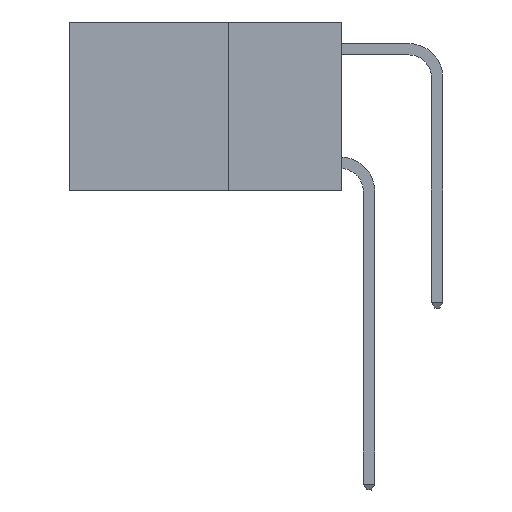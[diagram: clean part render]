
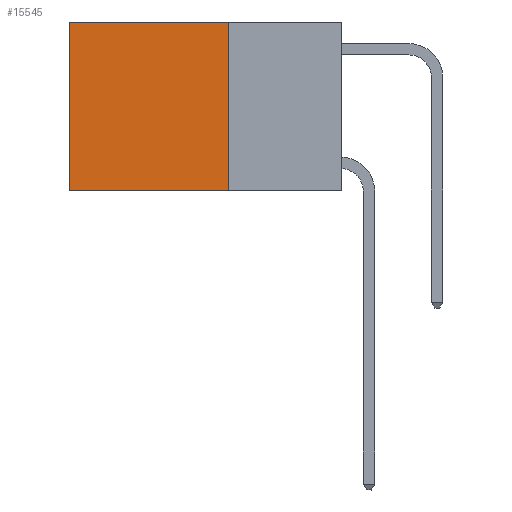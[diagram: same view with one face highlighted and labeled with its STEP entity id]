
A CAD part, left-side view. The second image highlights one B-rep face of the part: STEP entity #15545.
In plain terms, the highlighted planar face has unit normal (-1, 0, 0).
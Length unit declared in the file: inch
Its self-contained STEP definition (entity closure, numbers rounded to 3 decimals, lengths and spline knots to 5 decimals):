
#1530 = VECTOR ( 'NONE', #3508, 39.37008 ) ;
#3508 = DIRECTION ( 'NONE',  ( 0., 0., -1. ) ) ;
#3874 = EDGE_CURVE ( 'NONE', #4207, #9457, #12296, .T. ) ;
#4207 = VERTEX_POINT ( 'NONE', #15103 ) ;
#5973 = CARTESIAN_POINT ( 'NONE',  ( 0.2625, 0.25, 0. ) ) ;
#6600 = AXIS2_PLACEMENT_3D ( 'NONE', #9775, #12023, #27789 ) ;
#6822 = CARTESIAN_POINT ( 'NONE',  ( 0.2625, 0.6, 0. ) ) ;
#8485 = FACE_OUTER_BOUND ( 'NONE', #18595, .T. ) ;
#9457 = VERTEX_POINT ( 'NONE', #6822 ) ;
#9775 = CARTESIAN_POINT ( 'NONE',  ( 0.2625, 0.25, 0. ) ) ;
#10378 = EDGE_CURVE ( 'NONE', #9457, #12412, #19596, .T. ) ;
#10769 = LINE ( 'NONE', #23659, #15364 ) ;
#11673 = CARTESIAN_POINT ( 'NONE',  ( 0.2625, 0.25, 0. ) ) ;
#12023 = DIRECTION ( 'NONE',  ( 1., 0., 0. ) ) ;
#12296 = LINE ( 'NONE', #11673, #24304 ) ;
#12398 = ORIENTED_EDGE ( 'NONE', *, *, #13010, .F. ) ;
#12408 = DIRECTION ( 'NONE',  ( 0., 1., 0. ) ) ;
#12412 = VERTEX_POINT ( 'NONE', #19362 ) ;
#13010 = EDGE_CURVE ( 'NONE', #18789, #12412, #10769, .T. ) ;
#13878 = ORIENTED_EDGE ( 'NONE', *, *, #18491, .F. ) ;
#15103 = CARTESIAN_POINT ( 'NONE',  ( 0.2625, 0.25, 0. ) ) ;
#15364 = VECTOR ( 'NONE', #12408, 39.37008 ) ;
#15545 = ADVANCED_FACE ( 'NONE', ( #8485 ), #23289, .F. ) ;
#18491 = EDGE_CURVE ( 'NONE', #4207, #18789, #22839, .T. ) ;
#18595 = EDGE_LOOP ( 'NONE', ( #27157, #12398, #13878, #22835 ) ) ;
#18789 = VERTEX_POINT ( 'NONE', #22736 ) ;
#19362 = CARTESIAN_POINT ( 'NONE',  ( 0.2625, 0.6, -0.37 ) ) ;
#19596 = LINE ( 'NONE', #28246, #1530 ) ;
#21783 = DIRECTION ( 'NONE',  ( 0., 0., -1. ) ) ;
#22736 = CARTESIAN_POINT ( 'NONE',  ( 0.2625, 0.25, -0.37 ) ) ;
#22835 = ORIENTED_EDGE ( 'NONE', *, *, #3874, .T. ) ;
#22839 = LINE ( 'NONE', #5973, #28087 ) ;
#23289 = PLANE ( 'NONE',  #6600 ) ;
#23659 = CARTESIAN_POINT ( 'NONE',  ( 0.2625, 0.25, -0.37 ) ) ;
#24304 = VECTOR ( 'NONE', #27433, 39.37008 ) ;
#27157 = ORIENTED_EDGE ( 'NONE', *, *, #10378, .T. ) ;
#27433 = DIRECTION ( 'NONE',  ( 0., 1., 0. ) ) ;
#27789 = DIRECTION ( 'NONE',  ( 0., 0., -1. ) ) ;
#28087 = VECTOR ( 'NONE', #21783, 39.37008 ) ;
#28246 = CARTESIAN_POINT ( 'NONE',  ( 0.2625, 0.6, 0. ) ) ;
